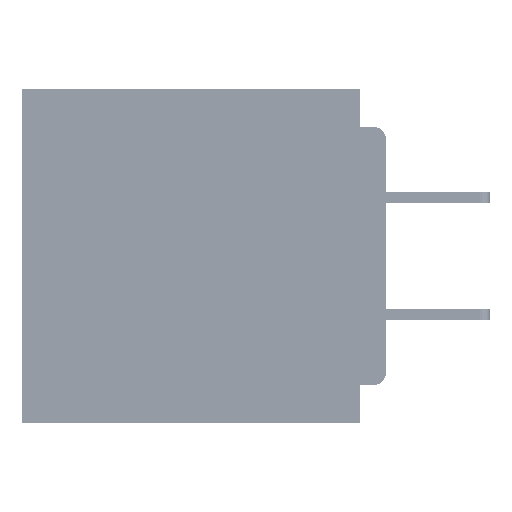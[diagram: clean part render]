
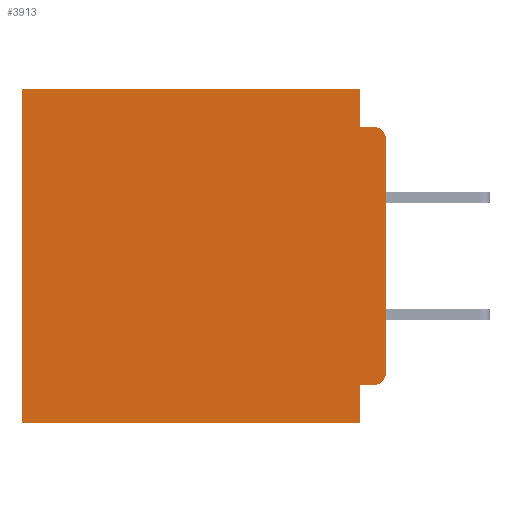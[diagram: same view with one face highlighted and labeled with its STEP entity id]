
A CAD part, left-side view. The second image highlights one B-rep face of the part: STEP entity #3913.
In plain terms, the highlighted planar face has unit normal (-1, 0, 0).
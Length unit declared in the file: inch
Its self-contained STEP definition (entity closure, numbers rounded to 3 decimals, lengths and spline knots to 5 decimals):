
#686 = ORIENTED_EDGE ( 'NONE', *, *, #62787, .F. ) ;
#1550 = CARTESIAN_POINT ( 'NONE',  ( 0.3, 0.031, -0.4 ) ) ;
#3913 = ADVANCED_FACE ( 'NONE', ( #13053 ), #22626, .F. ) ;
#5892 = ORIENTED_EDGE ( 'NONE', *, *, #42507, .F. ) ;
#6039 = LINE ( 'NONE', #42865, #32346 ) ;
#6892 = DIRECTION ( 'NONE',  ( 0., 0., -1. ) ) ;
#7495 = ORIENTED_EDGE ( 'NONE', *, *, #39891, .F. ) ;
#9150 = CARTESIAN_POINT ( 'NONE',  ( 0.3, 0., -0.045 ) ) ;
#9356 = VERTEX_POINT ( 'NONE', #57883 ) ;
#9394 = DIRECTION ( 'NONE',  ( -1., 0., 0. ) ) ;
#9771 = VECTOR ( 'NONE', #57522, 39.37008 ) ;
#9988 = CARTESIAN_POINT ( 'NONE',  ( 0.3, 0.031, 0. ) ) ;
#10731 = LINE ( 'NONE', #64109, #49274 ) ;
#11679 = DIRECTION ( 'NONE',  ( 0., 0., -1. ) ) ;
#13008 = ORIENTED_EDGE ( 'NONE', *, *, #60900, .F. ) ;
#13053 = FACE_OUTER_BOUND ( 'NONE', #23799, .T. ) ;
#13573 = VERTEX_POINT ( 'NONE', #51019 ) ;
#14406 = ORIENTED_EDGE ( 'NONE', *, *, #25868, .T. ) ;
#16721 = VERTEX_POINT ( 'NONE', #65418 ) ;
#18809 = CARTESIAN_POINT ( 'NONE',  ( 0.3, 0.015, -0.06 ) ) ;
#19630 = CARTESIAN_POINT ( 'NONE',  ( 0.3, 0.015, -0.355 ) ) ;
#19762 = VECTOR ( 'NONE', #6892, 39.37008 ) ;
#20841 = VECTOR ( 'NONE', #48785, 39.37008 ) ;
#20935 = ORIENTED_EDGE ( 'NONE', *, *, #49262, .T. ) ;
#21328 = VECTOR ( 'NONE', #11679, 39.37008 ) ;
#22626 = PLANE ( 'NONE',  #44046 ) ;
#23799 = EDGE_LOOP ( 'NONE', ( #50780, #20935, #65993, #5892, #14406, #29090, #13008, #7495, #686, #36802 ) ) ;
#24133 = DIRECTION ( 'NONE',  ( 0., 0., -1. ) ) ;
#25868 = EDGE_CURVE ( 'NONE', #54270, #46005, #37706, .T. ) ;
#26019 = CARTESIAN_POINT ( 'NONE',  ( 0.3, 0., 0. ) ) ;
#26320 = EDGE_CURVE ( 'NONE', #56402, #46836, #49887, .T. ) ;
#27932 = DIRECTION ( 'NONE',  ( 0., 0., -1. ) ) ;
#29090 = ORIENTED_EDGE ( 'NONE', *, *, #49146, .T. ) ;
#32346 = VECTOR ( 'NONE', #53387, 39.37008 ) ;
#33763 = LINE ( 'NONE', #53854, #19762 ) ;
#34235 = DIRECTION ( 'NONE',  ( 0., 1., 0. ) ) ;
#35070 = CARTESIAN_POINT ( 'NONE',  ( 0.3, 0.031, -0.045 ) ) ;
#36773 = LINE ( 'NONE', #60860, #49041 ) ;
#36802 = ORIENTED_EDGE ( 'NONE', *, *, #62981, .T. ) ;
#37636 = VECTOR ( 'NONE', #45823, 39.37008 ) ;
#37706 = LINE ( 'NONE', #26019, #9771 ) ;
#39891 = EDGE_CURVE ( 'NONE', #9356, #53876, #36773, .T. ) ;
#39978 = CARTESIAN_POINT ( 'NONE',  ( 0.3, 0.015, -0.045 ) ) ;
#40815 = CARTESIAN_POINT ( 'NONE',  ( 0.3, 0.015, -0.34 ) ) ;
#41276 = CIRCLE ( 'NONE', #42740, 0.015 ) ;
#42507 = EDGE_CURVE ( 'NONE', #54270, #56402, #33763, .T. ) ;
#42666 = CIRCLE ( 'NONE', #45562, 0.015 ) ;
#42740 = AXIS2_PLACEMENT_3D ( 'NONE', #18809, #55435, #24133 ) ;
#42865 = CARTESIAN_POINT ( 'NONE',  ( 0.3, 0.437, -0.4 ) ) ;
#44046 = AXIS2_PLACEMENT_3D ( 'NONE', #48723, #59196, #27932 ) ;
#45418 = LINE ( 'NONE', #59250, #20841 ) ;
#45562 = AXIS2_PLACEMENT_3D ( 'NONE', #40815, #9394, #46075 ) ;
#45823 = DIRECTION ( 'NONE',  ( 0., -1., 0. ) ) ;
#46005 = VERTEX_POINT ( 'NONE', #56569 ) ;
#46075 = DIRECTION ( 'NONE',  ( 0., 0., -1. ) ) ;
#46086 = VERTEX_POINT ( 'NONE', #46783 ) ;
#46783 = CARTESIAN_POINT ( 'NONE',  ( 0.3, 0., -0.34 ) ) ;
#46836 = VERTEX_POINT ( 'NONE', #39978 ) ;
#48723 = CARTESIAN_POINT ( 'NONE',  ( 0.3, 0., -0.4 ) ) ;
#48785 = DIRECTION ( 'NONE',  ( 0., 1., 0. ) ) ;
#49041 = VECTOR ( 'NONE', #61077, 39.37008 ) ;
#49146 = EDGE_CURVE ( 'NONE', #46005, #16721, #6039, .T. ) ;
#49262 = EDGE_CURVE ( 'NONE', #13573, #46836, #41276, .T. ) ;
#49274 = VECTOR ( 'NONE', #34235, 39.37008 ) ;
#49887 = LINE ( 'NONE', #9150, #37636 ) ;
#50163 = VERTEX_POINT ( 'NONE', #19630 ) ;
#50780 = ORIENTED_EDGE ( 'NONE', *, *, #63277, .F. ) ;
#51019 = CARTESIAN_POINT ( 'NONE',  ( 0.3, 0., -0.06 ) ) ;
#53387 = DIRECTION ( 'NONE',  ( 0., 0., -1. ) ) ;
#53854 = CARTESIAN_POINT ( 'NONE',  ( 0.3, 0.031, 0. ) ) ;
#53876 = VERTEX_POINT ( 'NONE', #1550 ) ;
#54270 = VERTEX_POINT ( 'NONE', #9988 ) ;
#55435 = DIRECTION ( 'NONE',  ( -1., 0., 0. ) ) ;
#56402 = VERTEX_POINT ( 'NONE', #35070 ) ;
#56569 = CARTESIAN_POINT ( 'NONE',  ( 0.3, 0.437, 0. ) ) ;
#57522 = DIRECTION ( 'NONE',  ( 0., 1., 0. ) ) ;
#57883 = CARTESIAN_POINT ( 'NONE',  ( 0.3, 0.031, -0.355 ) ) ;
#58809 = CARTESIAN_POINT ( 'NONE',  ( 0.3, 0., -0.4 ) ) ;
#59196 = DIRECTION ( 'NONE',  ( 1., 0., 0. ) ) ;
#59250 = CARTESIAN_POINT ( 'NONE',  ( 0.3, 0., -0.4 ) ) ;
#60860 = CARTESIAN_POINT ( 'NONE',  ( 0.3, 0.031, -0.4 ) ) ;
#60900 = EDGE_CURVE ( 'NONE', #53876, #16721, #45418, .T. ) ;
#61077 = DIRECTION ( 'NONE',  ( 0., 0., -1. ) ) ;
#61380 = LINE ( 'NONE', #58809, #21328 ) ;
#62787 = EDGE_CURVE ( 'NONE', #50163, #9356, #10731, .T. ) ;
#62981 = EDGE_CURVE ( 'NONE', #50163, #46086, #42666, .T. ) ;
#63277 = EDGE_CURVE ( 'NONE', #13573, #46086, #61380, .T. ) ;
#64109 = CARTESIAN_POINT ( 'NONE',  ( 0.3, 0., -0.355 ) ) ;
#65418 = CARTESIAN_POINT ( 'NONE',  ( 0.3, 0.437, -0.4 ) ) ;
#65993 = ORIENTED_EDGE ( 'NONE', *, *, #26320, .F. ) ;
